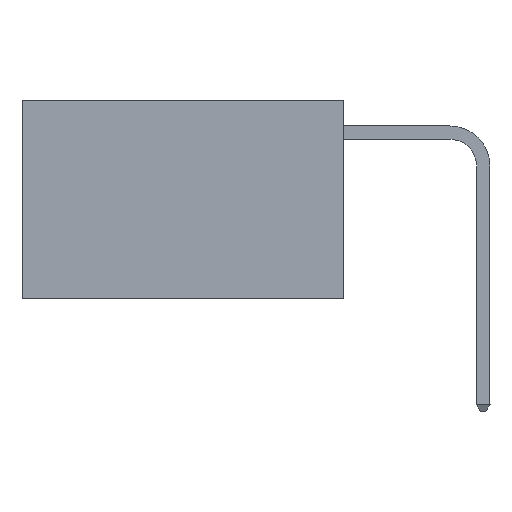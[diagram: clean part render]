
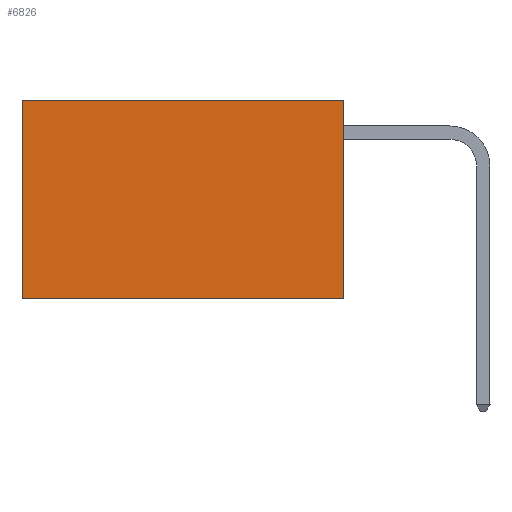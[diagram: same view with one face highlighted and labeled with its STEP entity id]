
A CAD part, left-side view. The second image highlights one B-rep face of the part: STEP entity #6826.
In plain terms, the highlighted planar face has unit normal (-1, 0, 0).
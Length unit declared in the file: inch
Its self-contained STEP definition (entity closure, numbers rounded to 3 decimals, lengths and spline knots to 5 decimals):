
#201 = CARTESIAN_POINT ( 'NONE',  ( 0.2625, 0., 0. ) ) ;
#549 = VERTEX_POINT ( 'NONE', #6164 ) ;
#861 = CARTESIAN_POINT ( 'NONE',  ( 0.2625, 0.6, -0.37 ) ) ;
#1371 = LINE ( 'NONE', #7630, #10449 ) ;
#1518 = DIRECTION ( 'NONE',  ( 0., 1., 0. ) ) ;
#2115 = VECTOR ( 'NONE', #1518, 39.37008 ) ;
#2140 = DIRECTION ( 'NONE',  ( 0., 1., 0. ) ) ;
#2857 = DIRECTION ( 'NONE',  ( 0., 0., -1. ) ) ;
#2868 = CARTESIAN_POINT ( 'NONE',  ( 0.2625, 0.6, 0. ) ) ;
#3063 = FACE_OUTER_BOUND ( 'NONE', #3900, .T. ) ;
#3663 = VECTOR ( 'NONE', #4803, 39.37008 ) ;
#3900 = EDGE_LOOP ( 'NONE', ( #4254, #9509, #9172, #5613 ) ) ;
#3945 = LINE ( 'NONE', #3951, #3663 ) ;
#3951 = CARTESIAN_POINT ( 'NONE',  ( 0.2625, 0., 0. ) ) ;
#4024 = EDGE_CURVE ( 'NONE', #549, #10548, #4450, .T. ) ;
#4154 = DIRECTION ( 'NONE',  ( 0., 0., -1. ) ) ;
#4254 = ORIENTED_EDGE ( 'NONE', *, *, #5359, .T. ) ;
#4450 = LINE ( 'NONE', #11399, #2115 ) ;
#4803 = DIRECTION ( 'NONE',  ( 0., 0., -1. ) ) ;
#5359 = EDGE_CURVE ( 'NONE', #9847, #10548, #9663, .T. ) ;
#5613 = ORIENTED_EDGE ( 'NONE', *, *, #5797, .T. ) ;
#5797 = EDGE_CURVE ( 'NONE', #8686, #9847, #1371, .T. ) ;
#6164 = CARTESIAN_POINT ( 'NONE',  ( 0.2625, 0., -0.37 ) ) ;
#6826 = ADVANCED_FACE ( 'NONE', ( #3063 ), #10990, .F. ) ;
#6924 = CARTESIAN_POINT ( 'NONE',  ( 0.2625, 0.6, 0. ) ) ;
#7235 = VECTOR ( 'NONE', #4154, 39.37008 ) ;
#7630 = CARTESIAN_POINT ( 'NONE',  ( 0.2625, 0., 0. ) ) ;
#8415 = DIRECTION ( 'NONE',  ( 1., 0., 0. ) ) ;
#8686 = VERTEX_POINT ( 'NONE', #11358 ) ;
#9172 = ORIENTED_EDGE ( 'NONE', *, *, #10061, .F. ) ;
#9509 = ORIENTED_EDGE ( 'NONE', *, *, #4024, .F. ) ;
#9663 = LINE ( 'NONE', #6924, #7235 ) ;
#9847 = VERTEX_POINT ( 'NONE', #2868 ) ;
#10061 = EDGE_CURVE ( 'NONE', #8686, #549, #3945, .T. ) ;
#10449 = VECTOR ( 'NONE', #2140, 39.37008 ) ;
#10548 = VERTEX_POINT ( 'NONE', #861 ) ;
#10990 = PLANE ( 'NONE',  #11088 ) ;
#11088 = AXIS2_PLACEMENT_3D ( 'NONE', #201, #8415, #2857 ) ;
#11358 = CARTESIAN_POINT ( 'NONE',  ( 0.2625, 0., 0. ) ) ;
#11399 = CARTESIAN_POINT ( 'NONE',  ( 0.2625, 0., -0.37 ) ) ;
